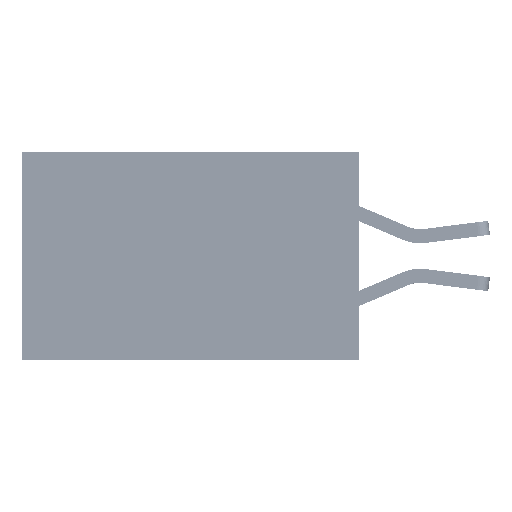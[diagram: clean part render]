
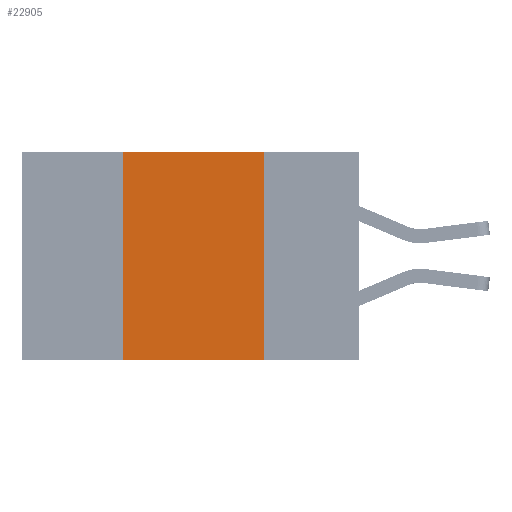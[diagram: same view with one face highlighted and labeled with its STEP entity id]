
A CAD part, left-side view. The second image highlights one B-rep face of the part: STEP entity #22905.
In plain terms, the highlighted planar face has unit normal (-1, 0, 0).
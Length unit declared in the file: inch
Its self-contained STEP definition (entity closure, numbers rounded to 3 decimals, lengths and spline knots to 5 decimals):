
#1541 = AXIS2_PLACEMENT_3D ( 'NONE', #2475, #2616, #9818 ) ;
#2475 = CARTESIAN_POINT ( 'NONE',  ( 0., 0.6, 0. ) ) ;
#2616 = DIRECTION ( 'NONE',  ( 1., 0., 0. ) ) ;
#4285 = CARTESIAN_POINT ( 'NONE',  ( 0., 0.17, 0. ) ) ;
#5156 = VECTOR ( 'NONE', #29791, 39.37008 ) ;
#8275 = ORIENTED_EDGE ( 'NONE', *, *, #13279, .T. ) ;
#9686 = CARTESIAN_POINT ( 'NONE',  ( 0., 0.17, -0.37 ) ) ;
#9818 = DIRECTION ( 'NONE',  ( 0., 0., -1. ) ) ;
#10697 = LINE ( 'NONE', #17810, #28154 ) ;
#13000 = LINE ( 'NONE', #4285, #5156 ) ;
#13205 = CARTESIAN_POINT ( 'NONE',  ( 0., 0.17, 0. ) ) ;
#13279 = EDGE_CURVE ( 'NONE', #32179, #39632, #10697, .T. ) ;
#13685 = DIRECTION ( 'NONE',  ( 0., 0., 1. ) ) ;
#13755 = EDGE_LOOP ( 'NONE', ( #42363, #31619, #25158, #8275 ) ) ;
#14314 = VECTOR ( 'NONE', #45872, 39.37008 ) ;
#17168 = CARTESIAN_POINT ( 'NONE',  ( 0., 0.6, 0. ) ) ;
#17810 = CARTESIAN_POINT ( 'NONE',  ( 0., 0.6, -0.37 ) ) ;
#18885 = EDGE_CURVE ( 'NONE', #32179, #29244, #40824, .T. ) ;
#20295 = EDGE_CURVE ( 'NONE', #29244, #20862, #38930, .T. ) ;
#20862 = VERTEX_POINT ( 'NONE', #13205 ) ;
#21774 = VECTOR ( 'NONE', #13685, 39.37008 ) ;
#22905 = ADVANCED_FACE ( 'NONE', ( #45928 ), #34226, .F. ) ;
#25158 = ORIENTED_EDGE ( 'NONE', *, *, #18885, .F. ) ;
#28154 = VECTOR ( 'NONE', #43202, 39.37008 ) ;
#29244 = VERTEX_POINT ( 'NONE', #43648 ) ;
#29791 = DIRECTION ( 'NONE',  ( 0., 0., -1. ) ) ;
#31619 = ORIENTED_EDGE ( 'NONE', *, *, #20295, .F. ) ;
#32179 = VERTEX_POINT ( 'NONE', #40406 ) ;
#34226 = PLANE ( 'NONE',  #1541 ) ;
#38847 = EDGE_CURVE ( 'NONE', #20862, #39632, #13000, .T. ) ;
#38930 = LINE ( 'NONE', #17168, #14314 ) ;
#39632 = VERTEX_POINT ( 'NONE', #9686 ) ;
#40406 = CARTESIAN_POINT ( 'NONE',  ( 0., 0.42, -0.37 ) ) ;
#40824 = LINE ( 'NONE', #45666, #21774 ) ;
#42363 = ORIENTED_EDGE ( 'NONE', *, *, #38847, .F. ) ;
#43202 = DIRECTION ( 'NONE',  ( 0., -1., 0. ) ) ;
#43648 = CARTESIAN_POINT ( 'NONE',  ( 0., 0.42, 0. ) ) ;
#45666 = CARTESIAN_POINT ( 'NONE',  ( 0., 0.42, 0. ) ) ;
#45872 = DIRECTION ( 'NONE',  ( 0., -1., 0. ) ) ;
#45928 = FACE_OUTER_BOUND ( 'NONE', #13755, .T. ) ;
